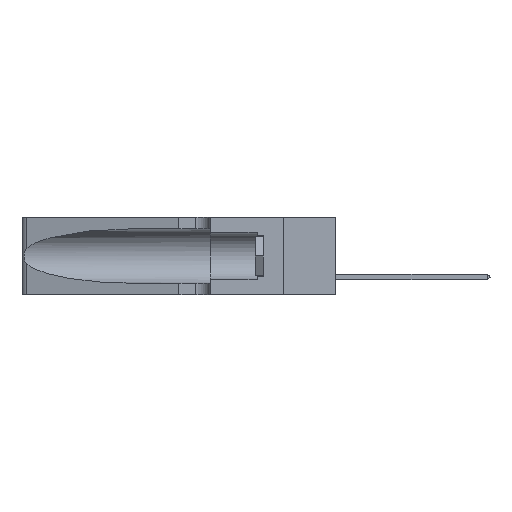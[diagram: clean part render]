
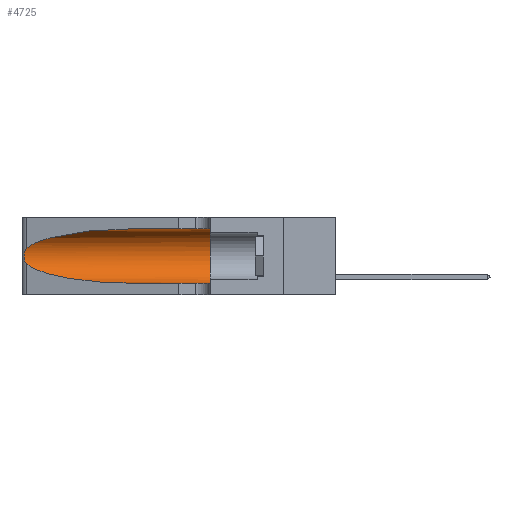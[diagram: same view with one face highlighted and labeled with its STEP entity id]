
A CAD part, left-side view. The second image highlights one B-rep face of the part: STEP entity #4725.
In plain terms, the highlighted cylindrical face has radius 3.308 mm (diameter 6.617 mm), a partial arc.
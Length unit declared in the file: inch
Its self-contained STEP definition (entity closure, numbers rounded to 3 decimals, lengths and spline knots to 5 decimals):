
#125 = ORIENTED_EDGE ( 'NONE', *, *, #1023, .F. ) ;
#633 = CARTESIAN_POINT ( 'NONE',  ( 0.25487, 1.22718, 0.22369 ) ) ;
#926 = VERTEX_POINT ( 'NONE', #36080 ) ;
#1023 = EDGE_CURVE ( 'NONE', #30504, #24860, #7624, .T. ) ;
#1380 = DIRECTION ( 'NONE',  ( 0., -1., 0. ) ) ;
#2274 =( BOUNDED_CURVE ( )  B_SPLINE_CURVE ( 3, ( #4601, #7782, #36401, #19028 ),
 .UNSPECIFIED., .F., .T. ) 
 B_SPLINE_CURVE_WITH_KNOTS ( ( 4, 4 ),
 ( 3.44316, 4.71239 ),
 .UNSPECIFIED. ) 
 CURVE ( )  GEOMETRIC_REPRESENTATION_ITEM ( )  RATIONAL_B_SPLINE_CURVE ( ( 1., 0.87, 0.87, 1. ) ) 
 REPRESENTATION_ITEM ( '' )  );
#2856 = CARTESIAN_POINT ( 'NONE',  ( 0.26075, 1.23896, 0.178 ) ) ;
#3423 = ORIENTED_EDGE ( 'NONE', *, *, #18904, .T. ) ;
#3721 = VERTEX_POINT ( 'NONE', #18864 ) ;
#3875 = CARTESIAN_POINT ( 'NONE',  ( 0.2373, 1.15595, 0.28018 ) ) ;
#4601 = CARTESIAN_POINT ( 'NONE',  ( 0.25487, 1.22718, 0.14631 ) ) ;
#4725 = ADVANCED_FACE ( 'NONE', ( #9303 ), #33833, .F. ) ;
#5245 = CARTESIAN_POINT ( 'NONE',  ( 0.26075, 1.23896, 0.19203 ) ) ;
#5495 = CARTESIAN_POINT ( 'NONE',  ( 0.25639, 1.23184, 0.21858 ) ) ;
#5616 = CARTESIAN_POINT ( 'NONE',  ( 0.25854, 1.2359, 0.20912 ) ) ;
#6082 = CARTESIAN_POINT ( 'NONE',  ( 0.1305, 0.35, 0.05475 ) ) ;
#7588 = CARTESIAN_POINT ( 'NONE',  ( 0.1305, 1.61858, 0.185 ) ) ;
#7624 = CIRCLE ( 'NONE', #13147, 0.13025 ) ;
#7782 = CARTESIAN_POINT ( 'NONE',  ( 0.2373, 1.15595, 0.08982 ) ) ;
#7944 = EDGE_CURVE ( 'NONE', #34901, #26198, #25187, .T. ) ;
#8429 = CARTESIAN_POINT ( 'NONE',  ( 0.25787, 1.23484, 0.2124 ) ) ;
#8682 = CARTESIAN_POINT ( 'NONE',  ( 0.25789, 1.23486, 0.15765 ) ) ;
#8747 = VECTOR ( 'NONE', #19064, 39.37008 ) ;
#9012 = AXIS2_PLACEMENT_3D ( 'NONE', #7588, #1380, #21923 ) ;
#9303 = FACE_OUTER_BOUND ( 'NONE', #13334, .T. ) ;
#11130 = CARTESIAN_POINT ( 'NONE',  ( 0.25555, 1.22993, 0.14849 ) ) ;
#11938 = ORIENTED_EDGE ( 'NONE', *, *, #37390, .T. ) ;
#13147 = AXIS2_PLACEMENT_3D ( 'NONE', #26648, #15650, #18495 ) ;
#13334 = EDGE_LOOP ( 'NONE', ( #11938, #25570, #35217, #3423, #125, #34703 ) ) ;
#14290 = CARTESIAN_POINT ( 'NONE',  ( 0.25639, 1.23186, 0.15144 ) ) ;
#15112 = LINE ( 'NONE', #34199, #8747 ) ;
#15650 = DIRECTION ( 'NONE',  ( 0., 1., 0. ) ) ;
#18495 = DIRECTION ( 'NONE',  ( 0., 0., 1. ) ) ;
#18864 = CARTESIAN_POINT ( 'NONE',  ( 0.1305, 0.72297, 0.31525 ) ) ;
#18904 = EDGE_CURVE ( 'NONE', #926, #24860, #33810, .T. ) ;
#19028 = CARTESIAN_POINT ( 'NONE',  ( 0.1305, 0.72297, 0.05475 ) ) ;
#19064 = DIRECTION ( 'NONE',  ( 0., -1., 0. ) ) ;
#19212 = CARTESIAN_POINT ( 'NONE',  ( 0.1305, 1.61858, 0.05475 ) ) ;
#19632 =( BOUNDED_CURVE ( )  B_SPLINE_CURVE ( 3, ( #35934, #30007, #3875, #27077 ),
 .UNSPECIFIED., .F., .T. ) 
 B_SPLINE_CURVE_WITH_KNOTS ( ( 4, 4 ),
 ( 1.5708, 2.84003 ),
 .UNSPECIFIED. ) 
 CURVE ( )  GEOMETRIC_REPRESENTATION_ITEM ( )  RATIONAL_B_SPLINE_CURVE ( ( 1., 0.87, 0.87, 1. ) ) 
 REPRESENTATION_ITEM ( '' )  );
#19772 = VECTOR ( 'NONE', #33143, 39.37008 ) ;
#20197 = CARTESIAN_POINT ( 'NONE',  ( 0.25555, 1.22994, 0.2215 ) ) ;
#21923 = DIRECTION ( 'NONE',  ( 0., 0., -1. ) ) ;
#22626 = CARTESIAN_POINT ( 'NONE',  ( 0.25487, 1.22718, 0.22369 ) ) ;
#24860 = VERTEX_POINT ( 'NONE', #6082 ) ;
#25187 = B_SPLINE_CURVE_WITH_KNOTS ( 'NONE', 3,
 ( #22626, #20197, #5495, #8429, #5616, #28485, #5245, #2856, #34525, #25654, #8682, #14290, #11130, #31389 ),
 .UNSPECIFIED., .F., .F.,
 ( 4, 2, 2, 2, 2, 2, 4 ),
 ( 0., 0.00027, 0.00053, 0.00107, 0.0016, 0.00187, 0.00214 ),
 .UNSPECIFIED. ) ;
#25570 = ORIENTED_EDGE ( 'NONE', *, *, #7944, .T. ) ;
#25654 = CARTESIAN_POINT ( 'NONE',  ( 0.25856, 1.23593, 0.16098 ) ) ;
#26198 = VERTEX_POINT ( 'NONE', #34405 ) ;
#26513 = CARTESIAN_POINT ( 'NONE',  ( 0.1305, 0.35, 0.31525 ) ) ;
#26648 = CARTESIAN_POINT ( 'NONE',  ( 0.1305, 0.35, 0.185 ) ) ;
#27077 = CARTESIAN_POINT ( 'NONE',  ( 0.25487, 1.22718, 0.22369 ) ) ;
#28485 = CARTESIAN_POINT ( 'NONE',  ( 0.26018, 1.23835, 0.19895 ) ) ;
#30007 = CARTESIAN_POINT ( 'NONE',  ( 0.18966, 0.96281, 0.31525 ) ) ;
#30504 = VERTEX_POINT ( 'NONE', #26513 ) ;
#31389 = CARTESIAN_POINT ( 'NONE',  ( 0.25487, 1.22718, 0.14631 ) ) ;
#33143 = DIRECTION ( 'NONE',  ( 0., -1., 0. ) ) ;
#33373 = EDGE_CURVE ( 'NONE', #3721, #30504, #15112, .T. ) ;
#33810 = LINE ( 'NONE', #19212, #19772 ) ;
#33833 = CYLINDRICAL_SURFACE ( 'NONE', #9012, 0.13025 ) ;
#34199 = CARTESIAN_POINT ( 'NONE',  ( 0.1305, 1.61858, 0.31525 ) ) ;
#34307 = EDGE_CURVE ( 'NONE', #26198, #926, #2274, .T. ) ;
#34405 = CARTESIAN_POINT ( 'NONE',  ( 0.25487, 1.22718, 0.14631 ) ) ;
#34525 = CARTESIAN_POINT ( 'NONE',  ( 0.26017, 1.23833, 0.17102 ) ) ;
#34703 = ORIENTED_EDGE ( 'NONE', *, *, #33373, .F. ) ;
#34901 = VERTEX_POINT ( 'NONE', #633 ) ;
#35217 = ORIENTED_EDGE ( 'NONE', *, *, #34307, .T. ) ;
#35934 = CARTESIAN_POINT ( 'NONE',  ( 0.1305, 0.72297, 0.31525 ) ) ;
#36080 = CARTESIAN_POINT ( 'NONE',  ( 0.1305, 0.72297, 0.05475 ) ) ;
#36401 = CARTESIAN_POINT ( 'NONE',  ( 0.18966, 0.96281, 0.05475 ) ) ;
#37390 = EDGE_CURVE ( 'NONE', #3721, #34901, #19632, .T. ) ;
